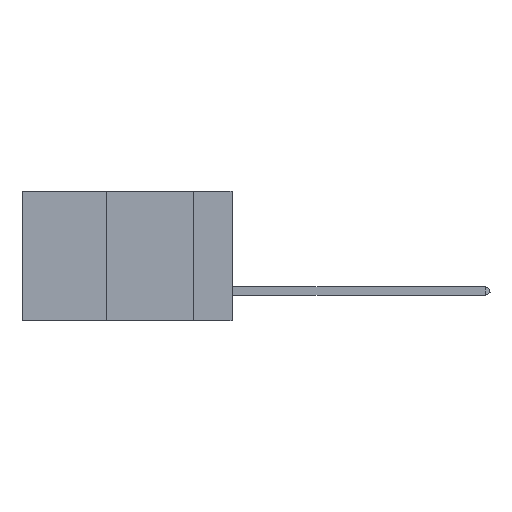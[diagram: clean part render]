
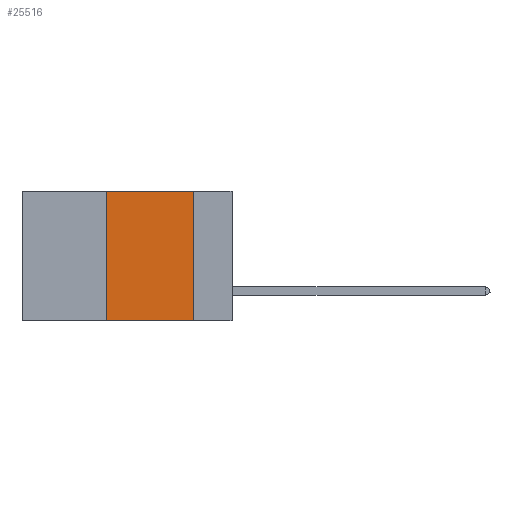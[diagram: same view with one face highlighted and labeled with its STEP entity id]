
A CAD part, left-side view. The second image highlights one B-rep face of the part: STEP entity #25516.
In plain terms, the highlighted planar face has unit normal (-1, 0, 0).
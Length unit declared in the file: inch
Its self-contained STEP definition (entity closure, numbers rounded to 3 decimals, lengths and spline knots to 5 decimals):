
#256 = VERTEX_POINT ( 'NONE', #45416 ) ;
#1455 = EDGE_CURVE ( 'NONE', #256, #9779, #38241, .T. ) ;
#2816 = EDGE_CURVE ( 'NONE', #34958, #19706, #2991, .T. ) ;
#2991 = LINE ( 'NONE', #5246, #33455 ) ;
#3599 = DIRECTION ( 'NONE',  ( 0., 0., 1. ) ) ;
#3620 = CARTESIAN_POINT ( 'NONE',  ( 0., 0.36, 0. ) ) ;
#4614 = AXIS2_PLACEMENT_3D ( 'NONE', #36436, #47934, #28474 ) ;
#5246 = CARTESIAN_POINT ( 'NONE',  ( 0., 0.11, 0. ) ) ;
#8263 = EDGE_LOOP ( 'NONE', ( #18599, #10473, #38545, #26073 ) ) ;
#9011 = DIRECTION ( 'NONE',  ( 0., 0., -1. ) ) ;
#9779 = VERTEX_POINT ( 'NONE', #3620 ) ;
#10265 = PLANE ( 'NONE',  #4614 ) ;
#10473 = ORIENTED_EDGE ( 'NONE', *, *, #16550, .F. ) ;
#14591 = CARTESIAN_POINT ( 'NONE',  ( 0., 0.6, 0. ) ) ;
#16454 = LINE ( 'NONE', #22424, #35147 ) ;
#16550 = EDGE_CURVE ( 'NONE', #9779, #34958, #21676, .T. ) ;
#18345 = CARTESIAN_POINT ( 'NONE',  ( 0., 0.36, 0. ) ) ;
#18599 = ORIENTED_EDGE ( 'NONE', *, *, #2816, .F. ) ;
#18730 = CARTESIAN_POINT ( 'NONE',  ( 0., 0.11, -0.37 ) ) ;
#19706 = VERTEX_POINT ( 'NONE', #18730 ) ;
#21676 = LINE ( 'NONE', #14591, #25217 ) ;
#22424 = CARTESIAN_POINT ( 'NONE',  ( 0., 0.6, -0.37 ) ) ;
#25217 = VECTOR ( 'NONE', #32740, 39.37008 ) ;
#25467 = EDGE_CURVE ( 'NONE', #256, #19706, #16454, .T. ) ;
#25516 = ADVANCED_FACE ( 'NONE', ( #35750 ), #10265, .F. ) ;
#26073 = ORIENTED_EDGE ( 'NONE', *, *, #25467, .T. ) ;
#28474 = DIRECTION ( 'NONE',  ( 0., 0., -1. ) ) ;
#28896 = VECTOR ( 'NONE', #3599, 39.37008 ) ;
#30157 = DIRECTION ( 'NONE',  ( 0., -1., 0. ) ) ;
#32740 = DIRECTION ( 'NONE',  ( 0., -1., 0. ) ) ;
#33455 = VECTOR ( 'NONE', #9011, 39.37008 ) ;
#34958 = VERTEX_POINT ( 'NONE', #43464 ) ;
#35147 = VECTOR ( 'NONE', #30157, 39.37008 ) ;
#35750 = FACE_OUTER_BOUND ( 'NONE', #8263, .T. ) ;
#36436 = CARTESIAN_POINT ( 'NONE',  ( 0., 0.6, 0. ) ) ;
#38241 = LINE ( 'NONE', #18345, #28896 ) ;
#38545 = ORIENTED_EDGE ( 'NONE', *, *, #1455, .F. ) ;
#43464 = CARTESIAN_POINT ( 'NONE',  ( 0., 0.11, 0. ) ) ;
#45416 = CARTESIAN_POINT ( 'NONE',  ( 0., 0.36, -0.37 ) ) ;
#47934 = DIRECTION ( 'NONE',  ( 1., 0., 0. ) ) ;
